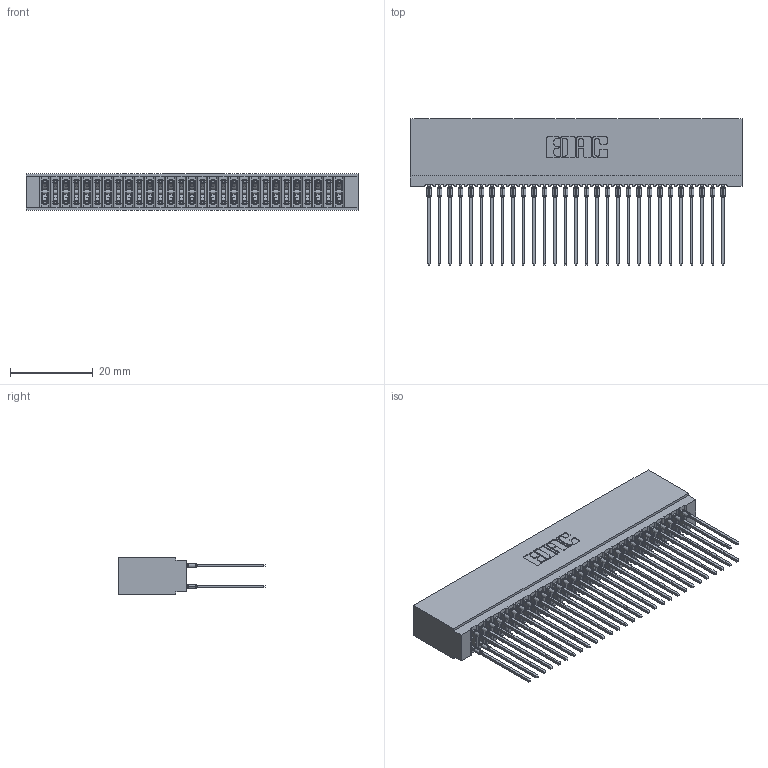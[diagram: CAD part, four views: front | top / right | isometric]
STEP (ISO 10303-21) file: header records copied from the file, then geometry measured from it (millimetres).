
FILE_DESCRIPTION (( 'STEP AP203' ), '1' );
FILE_NAME ('745-058-541-201.STEP', '2026-02-26T18:50:54', ( '' ), ( '' ), 'SwSTEP 2.0', 'SolidWorks 2023', '' );
FILE_SCHEMA (( 'CONFIG_CONTROL_DESIGN' ));
Length unit declared in the file: millimetre
Products named in the file (3): 745 Part_Insulator Option - 01; 745-292-001_541; 745-058-541-201
Assembly tree (59 placements, depth 2):
  745-058-541-201
    745 Part_Insulator Option - 01
    745-292-001_541  x58
Bounding box: 80.26 x 35.45 x 8.89 mm (x, y, z)
Volume: 7591.6 mm3; surface area: 16282.7 mm2
Topology: 59 solids, 59 shells, 5286 faces, 14207 edges, 8930 vertices
Faces by surface type: plane 2723, bspline 1160, cylinder 1055, torus 348
Entity records: 50597 total; most frequent: CARTESIAN_POINT 9283, ORIENTED_EDGE 8692, DIRECTION 7604, EDGE_CURVE 4346, VECTOR 3990, LINE 3990, VERTEX_POINT 2774, AXIS2_PLACEMENT_3D 1807
